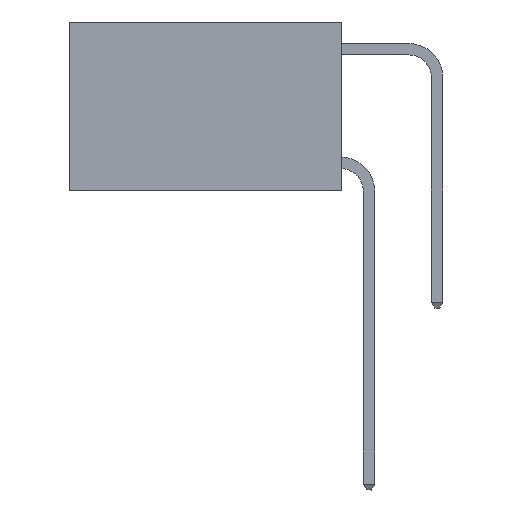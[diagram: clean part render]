
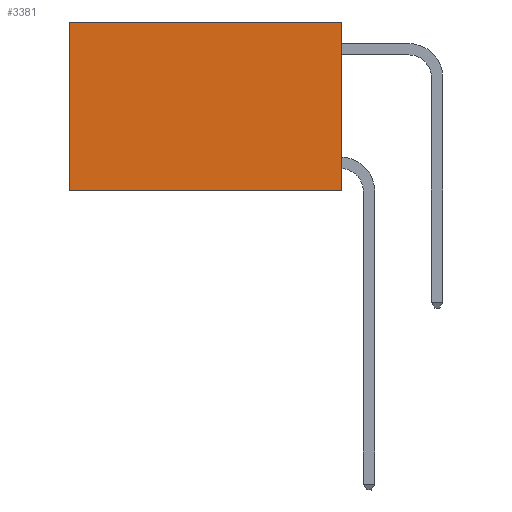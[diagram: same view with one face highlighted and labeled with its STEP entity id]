
A CAD part, left-side view. The second image highlights one B-rep face of the part: STEP entity #3381.
In plain terms, the highlighted planar face has unit normal (-1, 0, 0).
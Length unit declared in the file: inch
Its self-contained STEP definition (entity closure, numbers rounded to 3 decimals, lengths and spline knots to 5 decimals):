
#144 = VERTEX_POINT ( 'NONE', #1127 ) ;
#159 = ORIENTED_EDGE ( 'NONE', *, *, #19245, .T. ) ;
#282 = LINE ( 'NONE', #3379, #16501 ) ;
#506 = CARTESIAN_POINT ( 'NONE',  ( 0.2625, 0., -0.37 ) ) ;
#1127 = CARTESIAN_POINT ( 'NONE',  ( 0.2625, 0.6, -0.37 ) ) ;
#1473 = DIRECTION ( 'NONE',  ( 0., 0., -1. ) ) ;
#2223 = EDGE_CURVE ( 'NONE', #11969, #144, #6482, .T. ) ;
#3379 = CARTESIAN_POINT ( 'NONE',  ( 0.2625, 0., 0. ) ) ;
#3381 = ADVANCED_FACE ( 'NONE', ( #11804 ), #6253, .F. ) ;
#4504 = DIRECTION ( 'NONE',  ( 0., 0., -1. ) ) ;
#4869 = CARTESIAN_POINT ( 'NONE',  ( 0.2625, 0., -0.37 ) ) ;
#5442 = CARTESIAN_POINT ( 'NONE',  ( 0.2625, 0., 0. ) ) ;
#6253 = PLANE ( 'NONE',  #19326 ) ;
#6456 = DIRECTION ( 'NONE',  ( 0., 1., 0. ) ) ;
#6482 = LINE ( 'NONE', #15407, #10218 ) ;
#7729 = ORIENTED_EDGE ( 'NONE', *, *, #2223, .T. ) ;
#7884 = CARTESIAN_POINT ( 'NONE',  ( 0.2625, 0., 0. ) ) ;
#8215 = ORIENTED_EDGE ( 'NONE', *, *, #14928, .F. ) ;
#8898 = VERTEX_POINT ( 'NONE', #10910 ) ;
#9505 = LINE ( 'NONE', #4869, #17129 ) ;
#9700 = EDGE_CURVE ( 'NONE', #10847, #144, #9505, .T. ) ;
#10218 = VECTOR ( 'NONE', #4504, 39.37008 ) ;
#10847 = VERTEX_POINT ( 'NONE', #506 ) ;
#10910 = CARTESIAN_POINT ( 'NONE',  ( 0.2625, 0., 0. ) ) ;
#11010 = DIRECTION ( 'NONE',  ( 1., 0., 0. ) ) ;
#11804 = FACE_OUTER_BOUND ( 'NONE', #16567, .T. ) ;
#11969 = VERTEX_POINT ( 'NONE', #12069 ) ;
#12069 = CARTESIAN_POINT ( 'NONE',  ( 0.2625, 0.6, 0. ) ) ;
#14563 = VECTOR ( 'NONE', #14837, 39.37008 ) ;
#14837 = DIRECTION ( 'NONE',  ( 0., 1., 0. ) ) ;
#14928 = EDGE_CURVE ( 'NONE', #8898, #10847, #282, .T. ) ;
#15407 = CARTESIAN_POINT ( 'NONE',  ( 0.2625, 0.6, 0. ) ) ;
#15862 = DIRECTION ( 'NONE',  ( 0., 0., -1. ) ) ;
#15891 = ORIENTED_EDGE ( 'NONE', *, *, #9700, .F. ) ;
#16501 = VECTOR ( 'NONE', #15862, 39.37008 ) ;
#16567 = EDGE_LOOP ( 'NONE', ( #7729, #15891, #8215, #159 ) ) ;
#17129 = VECTOR ( 'NONE', #6456, 39.37008 ) ;
#18594 = LINE ( 'NONE', #5442, #14563 ) ;
#19245 = EDGE_CURVE ( 'NONE', #8898, #11969, #18594, .T. ) ;
#19326 = AXIS2_PLACEMENT_3D ( 'NONE', #7884, #11010, #1473 ) ;
